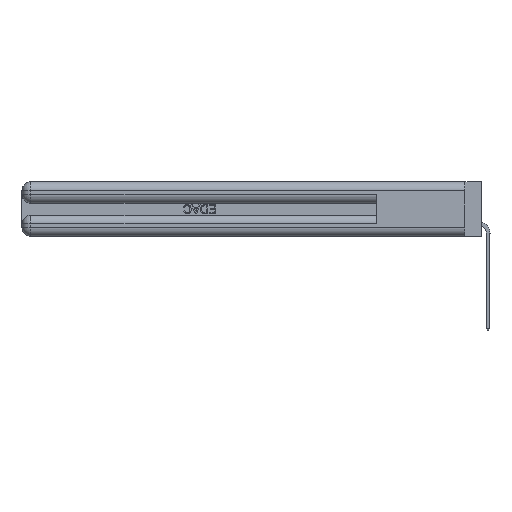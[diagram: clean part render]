
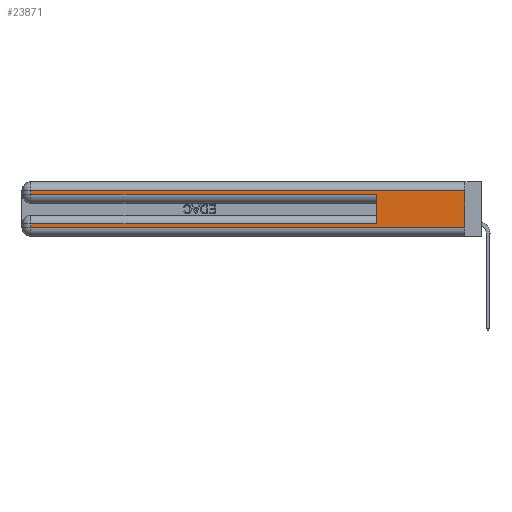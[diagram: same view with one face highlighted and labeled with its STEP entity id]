
A CAD part, left-side view. The second image highlights one B-rep face of the part: STEP entity #23871.
In plain terms, the highlighted planar face has unit normal (-1, 0, 0).
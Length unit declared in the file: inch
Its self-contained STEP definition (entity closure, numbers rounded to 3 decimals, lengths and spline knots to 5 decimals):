
#1442 = VECTOR ( 'NONE', #5847, 39.37008 ) ;
#2494 = VECTOR ( 'NONE', #15786, 39.37008 ) ;
#3899 = EDGE_CURVE ( 'NONE', #4067, #40263, #38227, .T. ) ;
#4067 = VERTEX_POINT ( 'NONE', #13923 ) ;
#4578 = EDGE_CURVE ( 'NONE', #40263, #27286, #26804, .T. ) ;
#5589 = ORIENTED_EDGE ( 'NONE', *, *, #45203, .F. ) ;
#5847 = DIRECTION ( 'NONE',  ( 0., 1., 0. ) ) ;
#7093 = EDGE_CURVE ( 'NONE', #27749, #36003, #9161, .T. ) ;
#8597 = CARTESIAN_POINT ( 'NONE',  ( 0., 0., 0.085 ) ) ;
#8699 = VERTEX_POINT ( 'NONE', #11326 ) ;
#9032 = ORIENTED_EDGE ( 'NONE', *, *, #42280, .T. ) ;
#9161 = LINE ( 'NONE', #15719, #17647 ) ;
#9313 = VECTOR ( 'NONE', #25917, 39.37008 ) ;
#11326 = CARTESIAN_POINT ( 'NONE',  ( 0., 0.6, 0.285 ) ) ;
#11427 = CARTESIAN_POINT ( 'NONE',  ( 0., 0., 0.06 ) ) ;
#13923 = CARTESIAN_POINT ( 'NONE',  ( 0., 0., 0.31 ) ) ;
#14210 = ORIENTED_EDGE ( 'NONE', *, *, #3899, .T. ) ;
#15371 = DIRECTION ( 'NONE',  ( 0., -1., 0. ) ) ;
#15719 = CARTESIAN_POINT ( 'NONE',  ( 0., 2.94, 0.37 ) ) ;
#15786 = DIRECTION ( 'NONE',  ( 0., 0., -1. ) ) ;
#16346 = ORIENTED_EDGE ( 'NONE', *, *, #24136, .F. ) ;
#16948 = CARTESIAN_POINT ( 'NONE',  ( 0., 2.94, 0.06 ) ) ;
#17647 = VECTOR ( 'NONE', #44812, 39.37008 ) ;
#17652 = VECTOR ( 'NONE', #38789, 39.37008 ) ;
#20916 = CARTESIAN_POINT ( 'NONE',  ( 0., 0., 0.06 ) ) ;
#21705 = VERTEX_POINT ( 'NONE', #24020 ) ;
#23217 = CARTESIAN_POINT ( 'NONE',  ( 0., 2.94, 0.37 ) ) ;
#23693 = DIRECTION ( 'NONE',  ( 0., -1., 0. ) ) ;
#23871 = ADVANCED_FACE ( 'NONE', ( #44346 ), #26038, .F. ) ;
#24020 = CARTESIAN_POINT ( 'NONE',  ( 0., 0.6, 0.085 ) ) ;
#24136 = EDGE_CURVE ( 'NONE', #4067, #41818, #39254, .T. ) ;
#24707 = EDGE_CURVE ( 'NONE', #21705, #27749, #44215, .T. ) ;
#25687 = VECTOR ( 'NONE', #23693, 39.37008 ) ;
#25917 = DIRECTION ( 'NONE',  ( 0., 0., 1. ) ) ;
#26038 = PLANE ( 'NONE',  #26288 ) ;
#26288 = AXIS2_PLACEMENT_3D ( 'NONE', #39511, #29829, #40451 ) ;
#26804 = LINE ( 'NONE', #23217, #2494 ) ;
#27279 = CARTESIAN_POINT ( 'NONE',  ( 0., 0., 0.37 ) ) ;
#27286 = VERTEX_POINT ( 'NONE', #31519 ) ;
#27614 = CARTESIAN_POINT ( 'NONE',  ( 0., 0., 0.285 ) ) ;
#27664 = CARTESIAN_POINT ( 'NONE',  ( 0., 0., 0.31 ) ) ;
#27749 = VERTEX_POINT ( 'NONE', #33858 ) ;
#29741 = EDGE_LOOP ( 'NONE', ( #16346, #14210, #39865, #9032, #5589, #38882, #42874, #43490 ) ) ;
#29829 = DIRECTION ( 'NONE',  ( 1., 0., 0. ) ) ;
#30071 = CARTESIAN_POINT ( 'NONE',  ( 0., 2.94, 0.31 ) ) ;
#31228 = DIRECTION ( 'NONE',  ( 0., 0., -1. ) ) ;
#31519 = CARTESIAN_POINT ( 'NONE',  ( 0., 2.94, 0.285 ) ) ;
#33858 = CARTESIAN_POINT ( 'NONE',  ( 0., 2.94, 0.085 ) ) ;
#35710 = EDGE_CURVE ( 'NONE', #36003, #41818, #41092, .T. ) ;
#36003 = VERTEX_POINT ( 'NONE', #16948 ) ;
#36833 = CARTESIAN_POINT ( 'NONE',  ( 0., 0.6, 0.145 ) ) ;
#36968 = LINE ( 'NONE', #27614, #25687 ) ;
#38227 = LINE ( 'NONE', #27664, #1442 ) ;
#38789 = DIRECTION ( 'NONE',  ( 0., 1., 0. ) ) ;
#38882 = ORIENTED_EDGE ( 'NONE', *, *, #24707, .T. ) ;
#39254 = LINE ( 'NONE', #27279, #44846 ) ;
#39511 = CARTESIAN_POINT ( 'NONE',  ( 0., 0., 0.37 ) ) ;
#39865 = ORIENTED_EDGE ( 'NONE', *, *, #4578, .T. ) ;
#39979 = VECTOR ( 'NONE', #15371, 39.37008 ) ;
#40263 = VERTEX_POINT ( 'NONE', #30071 ) ;
#40451 = DIRECTION ( 'NONE',  ( 0., 0., -1. ) ) ;
#41092 = LINE ( 'NONE', #11427, #39979 ) ;
#41818 = VERTEX_POINT ( 'NONE', #20916 ) ;
#42280 = EDGE_CURVE ( 'NONE', #27286, #8699, #36968, .T. ) ;
#42874 = ORIENTED_EDGE ( 'NONE', *, *, #7093, .T. ) ;
#43247 = LINE ( 'NONE', #36833, #9313 ) ;
#43490 = ORIENTED_EDGE ( 'NONE', *, *, #35710, .T. ) ;
#44215 = LINE ( 'NONE', #8597, #17652 ) ;
#44346 = FACE_OUTER_BOUND ( 'NONE', #29741, .T. ) ;
#44812 = DIRECTION ( 'NONE',  ( 0., 0., -1. ) ) ;
#44846 = VECTOR ( 'NONE', #31228, 39.37008 ) ;
#45203 = EDGE_CURVE ( 'NONE', #21705, #8699, #43247, .T. ) ;
